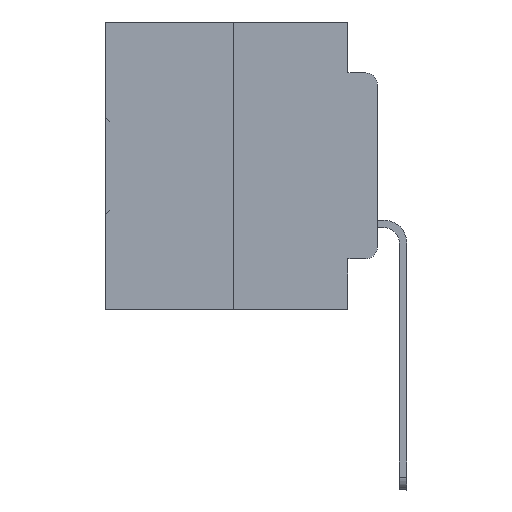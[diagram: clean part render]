
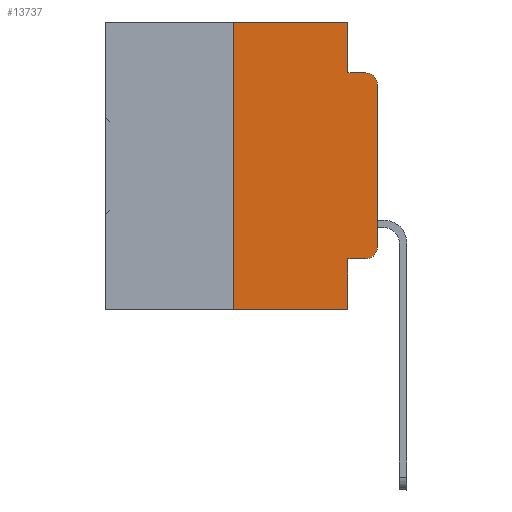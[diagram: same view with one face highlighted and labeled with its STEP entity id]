
A CAD part, left-side view. The second image highlights one B-rep face of the part: STEP entity #13737.
In plain terms, the highlighted planar face has unit normal (-1, 0, 0).
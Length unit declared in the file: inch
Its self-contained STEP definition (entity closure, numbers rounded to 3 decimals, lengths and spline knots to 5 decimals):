
#454 = LINE ( 'NONE', #30888, #17727 ) ;
#558 = ORIENTED_EDGE ( 'NONE', *, *, #28509, .F. ) ;
#1542 = CARTESIAN_POINT ( 'NONE',  ( 0., 0.25, 0. ) ) ;
#2474 = VERTEX_POINT ( 'NONE', #26814 ) ;
#2828 = LINE ( 'NONE', #10439, #24022 ) ;
#3071 = ORIENTED_EDGE ( 'NONE', *, *, #34140, .T. ) ;
#4376 = LINE ( 'NONE', #9452, #22677 ) ;
#4656 = CARTESIAN_POINT ( 'NONE',  ( 0., 0., -0.1085 ) ) ;
#5381 = VECTOR ( 'NONE', #21563, 39.37008 ) ;
#5383 = EDGE_LOOP ( 'NONE', ( #26586, #16133, #7592, #28871, #558, #19072, #22057, #28533, #10048, #3071 ) ) ;
#5530 = CARTESIAN_POINT ( 'NONE',  ( 0., 0.25, -0.5 ) ) ;
#6320 = LINE ( 'NONE', #27540, #30483 ) ;
#6412 = VERTEX_POINT ( 'NONE', #5530 ) ;
#7592 = ORIENTED_EDGE ( 'NONE', *, *, #22573, .F. ) ;
#8347 = LINE ( 'NONE', #10690, #5381 ) ;
#8403 = CARTESIAN_POINT ( 'NONE',  ( 0., 0.051, -0.5 ) ) ;
#8734 = LINE ( 'NONE', #27559, #18479 ) ;
#9452 = CARTESIAN_POINT ( 'NONE',  ( 0., 0.473, 0. ) ) ;
#9630 = DIRECTION ( 'NONE',  ( 0., -1., 0. ) ) ;
#10048 = ORIENTED_EDGE ( 'NONE', *, *, #17740, .T. ) ;
#10439 = CARTESIAN_POINT ( 'NONE',  ( 0., 0.25, 0. ) ) ;
#10690 = CARTESIAN_POINT ( 'NONE',  ( 0., 0.051, -0.4115 ) ) ;
#10703 = DIRECTION ( 'NONE',  ( 0., -1., 0. ) ) ;
#11077 = AXIS2_PLACEMENT_3D ( 'NONE', #17442, #30840, #17098 ) ;
#11515 = DIRECTION ( 'NONE',  ( 0., -1., 0. ) ) ;
#11624 = DIRECTION ( 'NONE',  ( 0., 0., -1. ) ) ;
#12099 = VERTEX_POINT ( 'NONE', #26494 ) ;
#12137 = PLANE ( 'NONE',  #15548 ) ;
#12802 = CARTESIAN_POINT ( 'NONE',  ( 0., 0., 0. ) ) ;
#13737 = ADVANCED_FACE ( 'NONE', ( #34035 ), #12137, .F. ) ;
#14487 = LINE ( 'NONE', #25516, #18051 ) ;
#15041 = DIRECTION ( 'NONE',  ( 0., 0., -1. ) ) ;
#15548 = AXIS2_PLACEMENT_3D ( 'NONE', #28425, #25907, #15041 ) ;
#16133 = ORIENTED_EDGE ( 'NONE', *, *, #16269, .T. ) ;
#16269 = EDGE_CURVE ( 'NONE', #19638, #2474, #35369, .T. ) ;
#17031 = VERTEX_POINT ( 'NONE', #1542 ) ;
#17098 = DIRECTION ( 'NONE',  ( 0., 0., -1. ) ) ;
#17442 = CARTESIAN_POINT ( 'NONE',  ( 0., 0.02, -0.1085 ) ) ;
#17484 = VECTOR ( 'NONE', #31986, 39.37008 ) ;
#17563 = DIRECTION ( 'NONE',  ( -1., 0., 0. ) ) ;
#17727 = VECTOR ( 'NONE', #11515, 39.37008 ) ;
#17740 = EDGE_CURVE ( 'NONE', #27802, #33673, #8347, .T. ) ;
#18051 = VECTOR ( 'NONE', #31476, 39.37008 ) ;
#18376 = VERTEX_POINT ( 'NONE', #20417 ) ;
#18479 = VECTOR ( 'NONE', #11624, 39.37008 ) ;
#19072 = ORIENTED_EDGE ( 'NONE', *, *, #19798, .F. ) ;
#19638 = VERTEX_POINT ( 'NONE', #4656 ) ;
#19798 = EDGE_CURVE ( 'NONE', #6412, #17031, #2828, .T. ) ;
#20417 = CARTESIAN_POINT ( 'NONE',  ( 0., 0.051, -0.0885 ) ) ;
#21563 = DIRECTION ( 'NONE',  ( 0., -1., 0. ) ) ;
#22057 = ORIENTED_EDGE ( 'NONE', *, *, #23331, .T. ) ;
#22573 = EDGE_CURVE ( 'NONE', #18376, #2474, #454, .T. ) ;
#22677 = VECTOR ( 'NONE', #9630, 39.37008 ) ;
#23160 = CARTESIAN_POINT ( 'NONE',  ( 0., 0.02, -0.3915 ) ) ;
#23310 = LINE ( 'NONE', #12802, #17484 ) ;
#23331 = EDGE_CURVE ( 'NONE', #6412, #24290, #6320, .T. ) ;
#24022 = VECTOR ( 'NONE', #24557, 39.37008 ) ;
#24195 = CARTESIAN_POINT ( 'NONE',  ( 0., 0.051, -0.4115 ) ) ;
#24290 = VERTEX_POINT ( 'NONE', #8403 ) ;
#24557 = DIRECTION ( 'NONE',  ( 0., 0., 1. ) ) ;
#25308 = EDGE_CURVE ( 'NONE', #12099, #18376, #8734, .T. ) ;
#25437 = CARTESIAN_POINT ( 'NONE',  ( 0., 0.02, -0.4115 ) ) ;
#25516 = CARTESIAN_POINT ( 'NONE',  ( 0., 0.051, 0. ) ) ;
#25907 = DIRECTION ( 'NONE',  ( 1., 0., 0. ) ) ;
#26358 = AXIS2_PLACEMENT_3D ( 'NONE', #23160, #17563, #28597 ) ;
#26494 = CARTESIAN_POINT ( 'NONE',  ( 0., 0.051, 0. ) ) ;
#26586 = ORIENTED_EDGE ( 'NONE', *, *, #30640, .T. ) ;
#26814 = CARTESIAN_POINT ( 'NONE',  ( 0., 0.02, -0.0885 ) ) ;
#27540 = CARTESIAN_POINT ( 'NONE',  ( 0., 0.473, -0.5 ) ) ;
#27559 = CARTESIAN_POINT ( 'NONE',  ( 0., 0.051, 0. ) ) ;
#27802 = VERTEX_POINT ( 'NONE', #24195 ) ;
#28425 = CARTESIAN_POINT ( 'NONE',  ( 0., 0.473, 0. ) ) ;
#28509 = EDGE_CURVE ( 'NONE', #17031, #12099, #4376, .T. ) ;
#28533 = ORIENTED_EDGE ( 'NONE', *, *, #28677, .F. ) ;
#28597 = DIRECTION ( 'NONE',  ( 0., 0., -1. ) ) ;
#28649 = CARTESIAN_POINT ( 'NONE',  ( 0., 0., -0.3915 ) ) ;
#28677 = EDGE_CURVE ( 'NONE', #27802, #24290, #14487, .T. ) ;
#28871 = ORIENTED_EDGE ( 'NONE', *, *, #25308, .F. ) ;
#30483 = VECTOR ( 'NONE', #10703, 39.37008 ) ;
#30640 = EDGE_CURVE ( 'NONE', #31464, #19638, #23310, .T. ) ;
#30840 = DIRECTION ( 'NONE',  ( -1., 0., 0. ) ) ;
#30888 = CARTESIAN_POINT ( 'NONE',  ( 0., 0.051, -0.0885 ) ) ;
#31464 = VERTEX_POINT ( 'NONE', #28649 ) ;
#31476 = DIRECTION ( 'NONE',  ( 0., 0., -1. ) ) ;
#31986 = DIRECTION ( 'NONE',  ( 0., 0., 1. ) ) ;
#33673 = VERTEX_POINT ( 'NONE', #25437 ) ;
#34035 = FACE_OUTER_BOUND ( 'NONE', #5383, .T. ) ;
#34140 = EDGE_CURVE ( 'NONE', #33673, #31464, #35029, .T. ) ;
#35029 = CIRCLE ( 'NONE', #26358, 0.02 ) ;
#35369 = CIRCLE ( 'NONE', #11077, 0.02 ) ;
